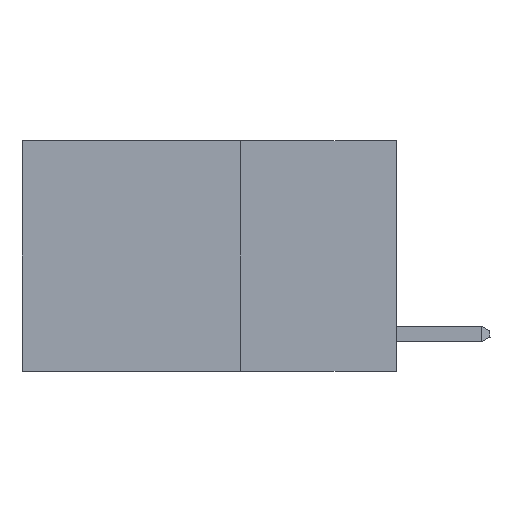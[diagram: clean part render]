
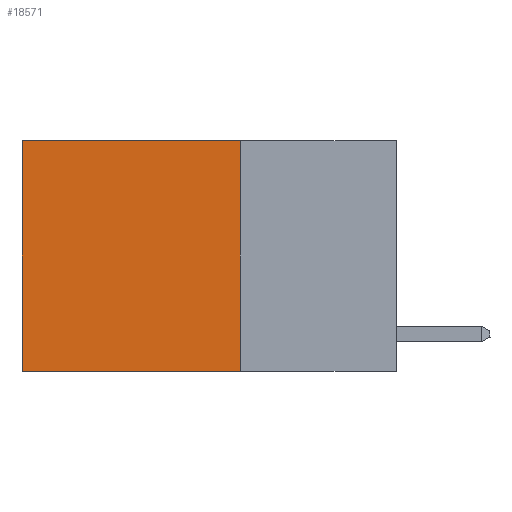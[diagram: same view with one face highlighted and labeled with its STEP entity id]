
A CAD part, left-side view. The second image highlights one B-rep face of the part: STEP entity #18571.
In plain terms, the highlighted planar face has unit normal (-1, 0, 0).
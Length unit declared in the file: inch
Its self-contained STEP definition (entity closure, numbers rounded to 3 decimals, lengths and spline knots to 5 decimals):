
#870 = VERTEX_POINT ( 'NONE', #3231 ) ;
#1615 = VERTEX_POINT ( 'NONE', #19763 ) ;
#2094 = ORIENTED_EDGE ( 'NONE', *, *, #15976, .T. ) ;
#2566 = CARTESIAN_POINT ( 'NONE',  ( 0.2625, 0.6, 0. ) ) ;
#2787 = CARTESIAN_POINT ( 'NONE',  ( 0.2625, 0.6, 0. ) ) ;
#3231 = CARTESIAN_POINT ( 'NONE',  ( 0.2625, 0.25, 0. ) ) ;
#3375 = ORIENTED_EDGE ( 'NONE', *, *, #10780, .T. ) ;
#4135 = DIRECTION ( 'NONE',  ( 0., 0., -1. ) ) ;
#4378 = VECTOR ( 'NONE', #6597, 39.37008 ) ;
#4905 = LINE ( 'NONE', #4939, #4378 ) ;
#4939 = CARTESIAN_POINT ( 'NONE',  ( 0.2625, 0.25, -0.37 ) ) ;
#5834 = ORIENTED_EDGE ( 'NONE', *, *, #13101, .F. ) ;
#6597 = DIRECTION ( 'NONE',  ( 0., 1., 0. ) ) ;
#6826 = VECTOR ( 'NONE', #12218, 39.37008 ) ;
#6850 = PLANE ( 'NONE',  #19161 ) ;
#6918 = CARTESIAN_POINT ( 'NONE',  ( 0.2625, 0.25, 0. ) ) ;
#8542 = DIRECTION ( 'NONE',  ( 0., 0., -1. ) ) ;
#10471 = ORIENTED_EDGE ( 'NONE', *, *, #19750, .F. ) ;
#10780 = EDGE_CURVE ( 'NONE', #18936, #11196, #19421, .T. ) ;
#11196 = VERTEX_POINT ( 'NONE', #14992 ) ;
#11961 = FACE_OUTER_BOUND ( 'NONE', #17317, .T. ) ;
#12118 = CARTESIAN_POINT ( 'NONE',  ( 0.2625, 0.25, 0. ) ) ;
#12218 = DIRECTION ( 'NONE',  ( 0., 0., -1. ) ) ;
#13101 = EDGE_CURVE ( 'NONE', #870, #1615, #16363, .T. ) ;
#13236 = DIRECTION ( 'NONE',  ( 0., 1., 0. ) ) ;
#14992 = CARTESIAN_POINT ( 'NONE',  ( 0.2625, 0.6, -0.37 ) ) ;
#15976 = EDGE_CURVE ( 'NONE', #870, #18936, #16008, .T. ) ;
#16008 = LINE ( 'NONE', #19501, #20173 ) ;
#16363 = LINE ( 'NONE', #12118, #20519 ) ;
#17317 = EDGE_LOOP ( 'NONE', ( #3375, #10471, #5834, #2094 ) ) ;
#18000 = DIRECTION ( 'NONE',  ( 1., 0., 0. ) ) ;
#18571 = ADVANCED_FACE ( 'NONE', ( #11961 ), #6850, .F. ) ;
#18936 = VERTEX_POINT ( 'NONE', #2787 ) ;
#19161 = AXIS2_PLACEMENT_3D ( 'NONE', #6918, #18000, #8542 ) ;
#19421 = LINE ( 'NONE', #2566, #6826 ) ;
#19501 = CARTESIAN_POINT ( 'NONE',  ( 0.2625, 0.25, 0. ) ) ;
#19750 = EDGE_CURVE ( 'NONE', #1615, #11196, #4905, .T. ) ;
#19763 = CARTESIAN_POINT ( 'NONE',  ( 0.2625, 0.25, -0.37 ) ) ;
#20173 = VECTOR ( 'NONE', #13236, 39.37008 ) ;
#20519 = VECTOR ( 'NONE', #4135, 39.37008 ) ;
